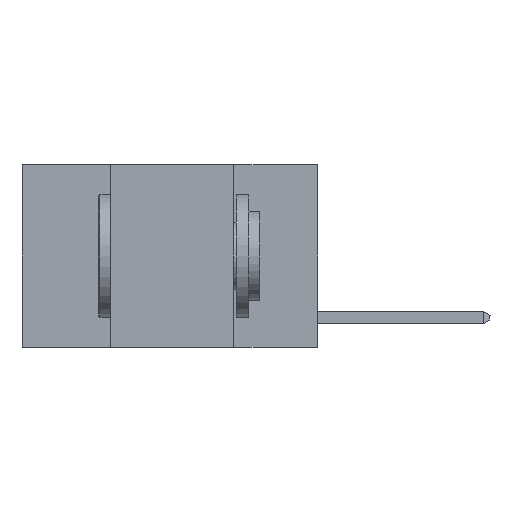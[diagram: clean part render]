
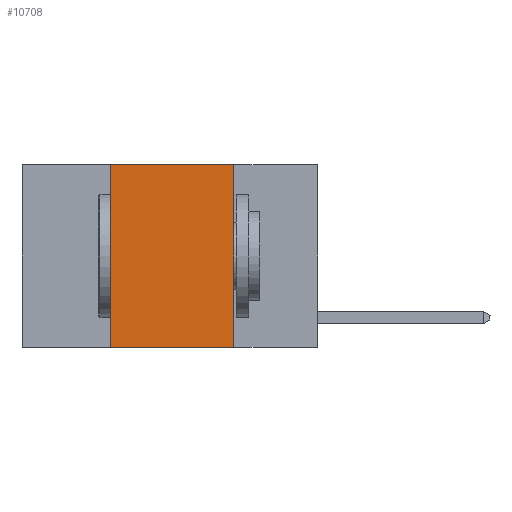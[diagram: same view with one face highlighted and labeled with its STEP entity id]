
A CAD part, left-side view. The second image highlights one B-rep face of the part: STEP entity #10708.
In plain terms, the highlighted planar face has unit normal (-1, 0, 0).
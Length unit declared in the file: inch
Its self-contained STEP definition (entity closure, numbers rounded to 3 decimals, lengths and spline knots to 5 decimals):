
#174 = EDGE_CURVE ( 'NONE', #10219, #1866, #3876, .T. ) ;
#603 = ORIENTED_EDGE ( 'NONE', *, *, #11394, .T. ) ;
#1866 = VERTEX_POINT ( 'NONE', #7414 ) ;
#1956 = LINE ( 'NONE', #2979, #9206 ) ;
#2006 = DIRECTION ( 'NONE',  ( 0., 0., -1. ) ) ;
#2553 = AXIS2_PLACEMENT_3D ( 'NONE', #5725, #7529, #2006 ) ;
#2577 = VERTEX_POINT ( 'NONE', #6426 ) ;
#2979 = CARTESIAN_POINT ( 'NONE',  ( 0., 0.42, 0. ) ) ;
#3458 = EDGE_CURVE ( 'NONE', #4542, #10219, #3523, .T. ) ;
#3523 = LINE ( 'NONE', #4289, #8006 ) ;
#3876 = LINE ( 'NONE', #5871, #8631 ) ;
#4289 = CARTESIAN_POINT ( 'NONE',  ( 0., 0.6, 0. ) ) ;
#4542 = VERTEX_POINT ( 'NONE', #6698 ) ;
#4618 = VECTOR ( 'NONE', #7171, 39.37008 ) ;
#4732 = ORIENTED_EDGE ( 'NONE', *, *, #3458, .F. ) ;
#5377 = ORIENTED_EDGE ( 'NONE', *, *, #11735, .F. ) ;
#5725 = CARTESIAN_POINT ( 'NONE',  ( 0., 0.6, 0. ) ) ;
#5871 = CARTESIAN_POINT ( 'NONE',  ( 0., 0.17, 0. ) ) ;
#5887 = EDGE_LOOP ( 'NONE', ( #8819, #4732, #5377, #603 ) ) ;
#6268 = CARTESIAN_POINT ( 'NONE',  ( 0., 0.6, -0.37 ) ) ;
#6426 = CARTESIAN_POINT ( 'NONE',  ( 0., 0.42, -0.37 ) ) ;
#6698 = CARTESIAN_POINT ( 'NONE',  ( 0., 0.42, 0. ) ) ;
#7171 = DIRECTION ( 'NONE',  ( 0., -1., 0. ) ) ;
#7414 = CARTESIAN_POINT ( 'NONE',  ( 0., 0.17, -0.37 ) ) ;
#7529 = DIRECTION ( 'NONE',  ( 1., 0., 0. ) ) ;
#8006 = VECTOR ( 'NONE', #8742, 39.37008 ) ;
#8631 = VECTOR ( 'NONE', #11490, 39.37008 ) ;
#8742 = DIRECTION ( 'NONE',  ( 0., -1., 0. ) ) ;
#8814 = CARTESIAN_POINT ( 'NONE',  ( 0., 0.17, 0. ) ) ;
#8819 = ORIENTED_EDGE ( 'NONE', *, *, #174, .F. ) ;
#9206 = VECTOR ( 'NONE', #9254, 39.37008 ) ;
#9254 = DIRECTION ( 'NONE',  ( 0., 0., 1. ) ) ;
#10152 = PLANE ( 'NONE',  #2553 ) ;
#10219 = VERTEX_POINT ( 'NONE', #8814 ) ;
#10353 = FACE_OUTER_BOUND ( 'NONE', #5887, .T. ) ;
#10708 = ADVANCED_FACE ( 'NONE', ( #10353 ), #10152, .F. ) ;
#11394 = EDGE_CURVE ( 'NONE', #2577, #1866, #11654, .T. ) ;
#11490 = DIRECTION ( 'NONE',  ( 0., 0., -1. ) ) ;
#11654 = LINE ( 'NONE', #6268, #4618 ) ;
#11735 = EDGE_CURVE ( 'NONE', #2577, #4542, #1956, .T. ) ;
